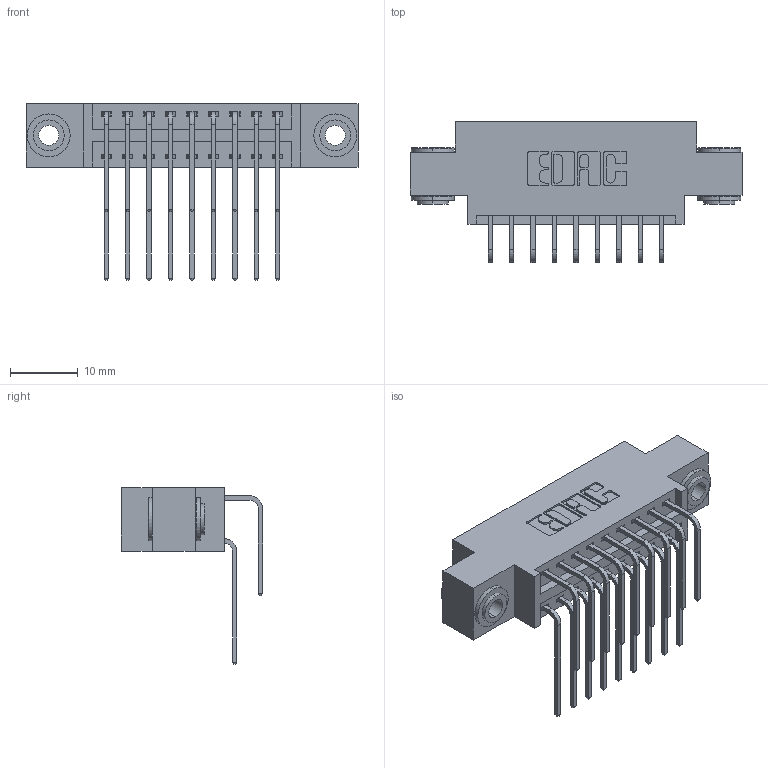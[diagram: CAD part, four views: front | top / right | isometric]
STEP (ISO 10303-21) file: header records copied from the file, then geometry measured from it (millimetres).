
FILE_DESCRIPTION (( 'STEP AP203' ), '1' );
FILE_NAME ('396-018-559-803.STEP', '2019-11-02T14:23:47', ( '' ), ( '' ), 'SwSTEP 2.0', 'SolidWorks 2016', '' );
FILE_SCHEMA (( 'CONFIG_CONTROL_DESIGN' ));
Length unit declared in the file: inch
Products named in the file (5): 396-018-559-803; 346 Part_0.170 Offset - 0.156 Dia-TH; 345-292-001_559 Tail - 2; 345-250-002_345-250-002-102; 345-292-001_558 559 Tail - 1
Assembly tree (21 placements, depth 2):
  396-018-559-803
    346 Part_0.170 Offset - 0.156 Dia-TH
    345-292-001_558 559 Tail - 1  x9
    345-292-001_559 Tail - 2  x9
    345-250-002_345-250-002-102  x2
Bounding box: 49.15 x 20.89 x 26.16 mm (x, y, z)
Volume: 4505 mm3; surface area: 6565.6 mm2
Topology: 21 solids, 21 shells, 1136 faces, 3315 edges, 2182 vertices
Faces by surface type: plane 756, cylinder 372, cone 8
Entity records: 12882 total; most frequent: CARTESIAN_POINT 2198, ORIENTED_EDGE 2074, DIRECTION 1991, EDGE_CURVE 1037, LINE 805, VECTOR 805, VERTEX_POINT 686, AXIS2_PLACEMENT_3D 593
